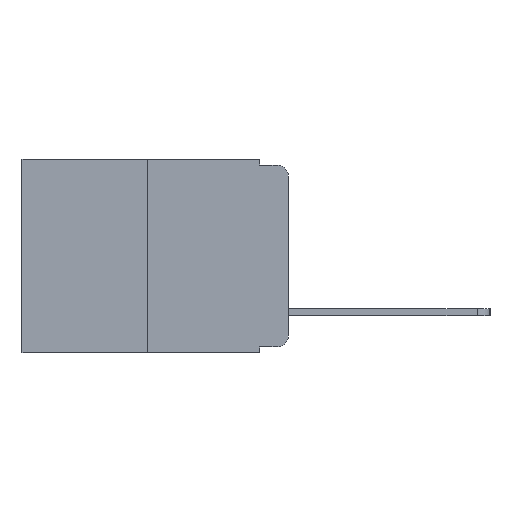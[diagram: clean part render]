
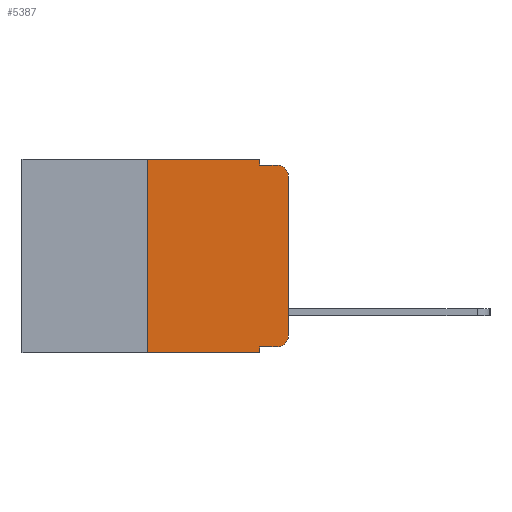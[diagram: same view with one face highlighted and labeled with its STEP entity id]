
A CAD part, left-side view. The second image highlights one B-rep face of the part: STEP entity #5387.
In plain terms, the highlighted planar face has unit normal (-1, 0, 0).
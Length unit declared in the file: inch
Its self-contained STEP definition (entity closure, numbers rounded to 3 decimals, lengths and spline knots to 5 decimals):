
#34 = VERTEX_POINT ( 'NONE', #8287 ) ;
#43 = EDGE_CURVE ( 'NONE', #9092, #2507, #808, .T. ) ;
#162 = CARTESIAN_POINT ( 'NONE',  ( 0., 0.25, 0. ) ) ;
#686 = DIRECTION ( 'NONE',  ( 0., 0., -1. ) ) ;
#752 = LINE ( 'NONE', #5538, #2759 ) ;
#808 = LINE ( 'NONE', #9946, #5194 ) ;
#847 = EDGE_CURVE ( 'NONE', #3306, #8690, #8574, .T. ) ;
#1081 = VERTEX_POINT ( 'NONE', #10920 ) ;
#1163 = VECTOR ( 'NONE', #8486, 39.37008 ) ;
#1364 = EDGE_CURVE ( 'NONE', #8690, #2975, #6661, .T. ) ;
#1437 = DIRECTION ( 'NONE',  ( -1., 0., 0. ) ) ;
#1547 = FACE_OUTER_BOUND ( 'NONE', #10801, .T. ) ;
#1590 = AXIS2_PLACEMENT_3D ( 'NONE', #3774, #1437, #10143 ) ;
#1663 = VECTOR ( 'NONE', #5748, 39.37008 ) ;
#1712 = LINE ( 'NONE', #6461, #4042 ) ;
#1718 = EDGE_CURVE ( 'NONE', #2507, #34, #10184, .T. ) ;
#2036 = CARTESIAN_POINT ( 'NONE',  ( 0., 0.051, -0.01 ) ) ;
#2158 = CARTESIAN_POINT ( 'NONE',  ( 0., 0.25, 0. ) ) ;
#2444 = CARTESIAN_POINT ( 'NONE',  ( 0., 0.051, -0.01 ) ) ;
#2507 = VERTEX_POINT ( 'NONE', #9076 ) ;
#2524 = CARTESIAN_POINT ( 'NONE',  ( 0., 0.051, 0. ) ) ;
#2681 = DIRECTION ( 'NONE',  ( 0., 0., 1. ) ) ;
#2759 = VECTOR ( 'NONE', #4663, 39.37008 ) ;
#2975 = VERTEX_POINT ( 'NONE', #2524 ) ;
#2984 = EDGE_CURVE ( 'NONE', #3306, #4616, #1712, .T. ) ;
#3126 = ORIENTED_EDGE ( 'NONE', *, *, #6642, .F. ) ;
#3306 = VERTEX_POINT ( 'NONE', #5623 ) ;
#3485 = LINE ( 'NONE', #8763, #1163 ) ;
#3494 = CARTESIAN_POINT ( 'NONE',  ( 0., 0.051, -0.343 ) ) ;
#3764 = EDGE_CURVE ( 'NONE', #9092, #4616, #3485, .T. ) ;
#3774 = CARTESIAN_POINT ( 'NONE',  ( 0., 0.02, -0.313 ) ) ;
#3974 = EDGE_CURVE ( 'NONE', #8540, #1081, #6233, .T. ) ;
#3988 = LINE ( 'NONE', #2036, #1663 ) ;
#4042 = VECTOR ( 'NONE', #6584, 39.37008 ) ;
#4259 = ORIENTED_EDGE ( 'NONE', *, *, #8076, .F. ) ;
#4282 = AXIS2_PLACEMENT_3D ( 'NONE', #4856, #5729, #686 ) ;
#4616 = VERTEX_POINT ( 'NONE', #3494 ) ;
#4663 = DIRECTION ( 'NONE',  ( 0., 0., 1. ) ) ;
#4856 = CARTESIAN_POINT ( 'NONE',  ( 0., 0.473, 0. ) ) ;
#4885 = VECTOR ( 'NONE', #6913, 39.37008 ) ;
#4928 = VECTOR ( 'NONE', #7173, 39.37008 ) ;
#5096 = ORIENTED_EDGE ( 'NONE', *, *, #847, .F. ) ;
#5194 = VECTOR ( 'NONE', #7530, 39.37008 ) ;
#5218 = DIRECTION ( 'NONE',  ( 0., 0., -1. ) ) ;
#5387 = ADVANCED_FACE ( 'NONE', ( #1547 ), #10896, .F. ) ;
#5538 = CARTESIAN_POINT ( 'NONE',  ( 0., 0., 0. ) ) ;
#5623 = CARTESIAN_POINT ( 'NONE',  ( 0., 0.25, -0.343 ) ) ;
#5729 = DIRECTION ( 'NONE',  ( 1., 0., 0. ) ) ;
#5748 = DIRECTION ( 'NONE',  ( 0., -1., 0. ) ) ;
#5917 = ORIENTED_EDGE ( 'NONE', *, *, #43, .T. ) ;
#6038 = ORIENTED_EDGE ( 'NONE', *, *, #3974, .T. ) ;
#6233 = CIRCLE ( 'NONE', #7135, 0.02 ) ;
#6260 = VECTOR ( 'NONE', #2681, 39.37008 ) ;
#6323 = ORIENTED_EDGE ( 'NONE', *, *, #3764, .F. ) ;
#6461 = CARTESIAN_POINT ( 'NONE',  ( 0., 0.473, -0.343 ) ) ;
#6584 = DIRECTION ( 'NONE',  ( 0., -1., 0. ) ) ;
#6642 = EDGE_CURVE ( 'NONE', #7803, #1081, #3988, .T. ) ;
#6661 = LINE ( 'NONE', #6951, #4885 ) ;
#6775 = CARTESIAN_POINT ( 'NONE',  ( 0., 0.051, -0.333 ) ) ;
#6913 = DIRECTION ( 'NONE',  ( 0., -1., 0. ) ) ;
#6951 = CARTESIAN_POINT ( 'NONE',  ( 0., 0.473, 0. ) ) ;
#7025 = ORIENTED_EDGE ( 'NONE', *, *, #1718, .T. ) ;
#7135 = AXIS2_PLACEMENT_3D ( 'NONE', #8899, #8123, #5218 ) ;
#7173 = DIRECTION ( 'NONE',  ( 0., 0., -1. ) ) ;
#7530 = DIRECTION ( 'NONE',  ( 0., -1., 0. ) ) ;
#7672 = ORIENTED_EDGE ( 'NONE', *, *, #9465, .T. ) ;
#7803 = VERTEX_POINT ( 'NONE', #2444 ) ;
#7824 = ORIENTED_EDGE ( 'NONE', *, *, #2984, .T. ) ;
#7944 = ORIENTED_EDGE ( 'NONE', *, *, #1364, .F. ) ;
#8076 = EDGE_CURVE ( 'NONE', #2975, #7803, #9820, .T. ) ;
#8123 = DIRECTION ( 'NONE',  ( -1., 0., 0. ) ) ;
#8287 = CARTESIAN_POINT ( 'NONE',  ( 0., 0., -0.313 ) ) ;
#8486 = DIRECTION ( 'NONE',  ( 0., 0., -1. ) ) ;
#8540 = VERTEX_POINT ( 'NONE', #11178 ) ;
#8574 = LINE ( 'NONE', #2158, #6260 ) ;
#8690 = VERTEX_POINT ( 'NONE', #162 ) ;
#8763 = CARTESIAN_POINT ( 'NONE',  ( 0., 0.051, 0. ) ) ;
#8899 = CARTESIAN_POINT ( 'NONE',  ( 0., 0.02, -0.03 ) ) ;
#9076 = CARTESIAN_POINT ( 'NONE',  ( 0., 0.02, -0.333 ) ) ;
#9092 = VERTEX_POINT ( 'NONE', #6775 ) ;
#9465 = EDGE_CURVE ( 'NONE', #34, #8540, #752, .T. ) ;
#9744 = CARTESIAN_POINT ( 'NONE',  ( 0., 0.051, 0. ) ) ;
#9820 = LINE ( 'NONE', #9744, #4928 ) ;
#9946 = CARTESIAN_POINT ( 'NONE',  ( 0., 0.051, -0.333 ) ) ;
#10143 = DIRECTION ( 'NONE',  ( 0., 0., -1. ) ) ;
#10184 = CIRCLE ( 'NONE', #1590, 0.02 ) ;
#10801 = EDGE_LOOP ( 'NONE', ( #7672, #6038, #3126, #4259, #7944, #5096, #7824, #6323, #5917, #7025 ) ) ;
#10896 = PLANE ( 'NONE',  #4282 ) ;
#10920 = CARTESIAN_POINT ( 'NONE',  ( 0., 0.02, -0.01 ) ) ;
#11178 = CARTESIAN_POINT ( 'NONE',  ( 0., 0., -0.03 ) ) ;
